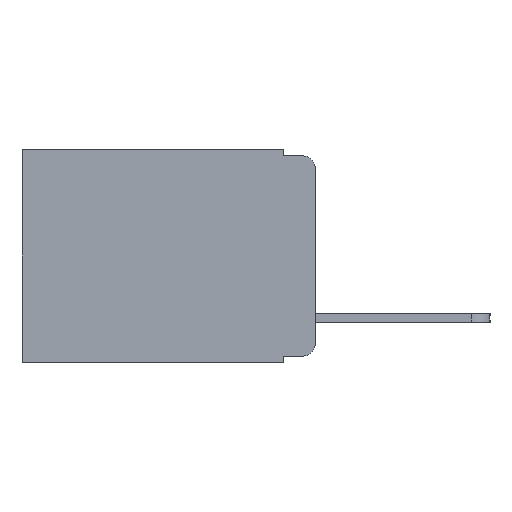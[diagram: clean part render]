
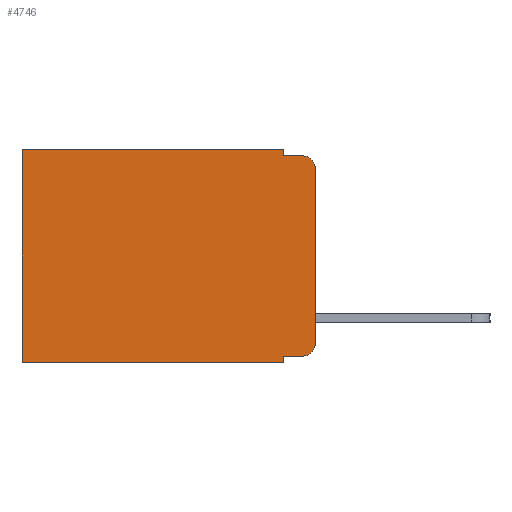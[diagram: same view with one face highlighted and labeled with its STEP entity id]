
A CAD part, left-side view. The second image highlights one B-rep face of the part: STEP entity #4746.
In plain terms, the highlighted planar face has unit normal (-1, 0, 0).
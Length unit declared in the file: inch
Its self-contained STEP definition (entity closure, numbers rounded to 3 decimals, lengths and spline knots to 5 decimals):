
#179 = CARTESIAN_POINT ( 'NONE',  ( 0.298, 0.02, -0.333 ) ) ;
#397 = EDGE_CURVE ( 'NONE', #7864, #15411, #7242, .T. ) ;
#453 = CARTESIAN_POINT ( 'NONE',  ( 0.298, 0.051, -0.333 ) ) ;
#801 = EDGE_CURVE ( 'NONE', #10526, #15889, #5974, .T. ) ;
#900 = VERTEX_POINT ( 'NONE', #15758 ) ;
#1177 = CARTESIAN_POINT ( 'NONE',  ( 0.298, 0., -0.313 ) ) ;
#1246 = VERTEX_POINT ( 'NONE', #7143 ) ;
#1386 = LINE ( 'NONE', #15184, #13645 ) ;
#1402 = CARTESIAN_POINT ( 'NONE',  ( 0.298, 0., 0. ) ) ;
#2351 = DIRECTION ( 'NONE',  ( 0., -1., 0. ) ) ;
#2799 = DIRECTION ( 'NONE',  ( 0., -1., 0. ) ) ;
#2894 = ORIENTED_EDGE ( 'NONE', *, *, #16190, .F. ) ;
#3100 = LINE ( 'NONE', #17560, #6743 ) ;
#3113 = CARTESIAN_POINT ( 'NONE',  ( 0.298, 0.051, -0.01 ) ) ;
#3884 = VERTEX_POINT ( 'NONE', #15283 ) ;
#4071 = EDGE_CURVE ( 'NONE', #10526, #7864, #5906, .T. ) ;
#4098 = CARTESIAN_POINT ( 'NONE',  ( 0.298, 0.473, 0. ) ) ;
#4107 = ORIENTED_EDGE ( 'NONE', *, *, #8979, .T. ) ;
#4514 = EDGE_LOOP ( 'NONE', ( #13406, #15881, #5519, #2894, #4107, #16439, #17451, #18480, #11206, #8338 ) ) ;
#4746 = ADVANCED_FACE ( 'NONE', ( #17765 ), #8177, .F. ) ;
#5051 = DIRECTION ( 'NONE',  ( -1., 0., 0. ) ) ;
#5519 = ORIENTED_EDGE ( 'NONE', *, *, #10094, .F. ) ;
#5906 = LINE ( 'NONE', #453, #14370 ) ;
#5921 = DIRECTION ( 'NONE',  ( 0., 0., -1. ) ) ;
#5974 = LINE ( 'NONE', #16728, #17634 ) ;
#6006 = LINE ( 'NONE', #3113, #10203 ) ;
#6701 = DIRECTION ( 'NONE',  ( 0., 1., 0. ) ) ;
#6743 = VECTOR ( 'NONE', #18883, 39.37008 ) ;
#7053 = EDGE_CURVE ( 'NONE', #15889, #7070, #11184, .T. ) ;
#7070 = VERTEX_POINT ( 'NONE', #11303 ) ;
#7143 = CARTESIAN_POINT ( 'NONE',  ( 0.298, 0.051, -0.01 ) ) ;
#7199 = AXIS2_PLACEMENT_3D ( 'NONE', #16201, #5051, #13445 ) ;
#7242 = CIRCLE ( 'NONE', #7199, 0.02 ) ;
#7453 = VERTEX_POINT ( 'NONE', #11986 ) ;
#7864 = VERTEX_POINT ( 'NONE', #179 ) ;
#8177 = PLANE ( 'NONE',  #19312 ) ;
#8287 = CARTESIAN_POINT ( 'NONE',  ( 0.298, 0.051, 0. ) ) ;
#8338 = ORIENTED_EDGE ( 'NONE', *, *, #397, .T. ) ;
#8865 = CARTESIAN_POINT ( 'NONE',  ( 0.298, 0.02, -0.03 ) ) ;
#8926 = CARTESIAN_POINT ( 'NONE',  ( 0.298, 0., 0. ) ) ;
#8979 = EDGE_CURVE ( 'NONE', #17239, #3884, #1386, .T. ) ;
#9280 = CARTESIAN_POINT ( 'NONE',  ( 0.298, 0., -0.343 ) ) ;
#9281 = DIRECTION ( 'NONE',  ( 0., 0., -1. ) ) ;
#9441 = AXIS2_PLACEMENT_3D ( 'NONE', #8865, #18719, #10402 ) ;
#10094 = EDGE_CURVE ( 'NONE', #1246, #900, #6006, .T. ) ;
#10203 = VECTOR ( 'NONE', #2351, 39.37008 ) ;
#10402 = DIRECTION ( 'NONE',  ( 0., 0., -1. ) ) ;
#10526 = VERTEX_POINT ( 'NONE', #12704 ) ;
#10699 = VECTOR ( 'NONE', #11778, 39.37008 ) ;
#11184 = LINE ( 'NONE', #9280, #10699 ) ;
#11206 = ORIENTED_EDGE ( 'NONE', *, *, #4071, .T. ) ;
#11303 = CARTESIAN_POINT ( 'NONE',  ( 0.298, 0.473, -0.343 ) ) ;
#11778 = DIRECTION ( 'NONE',  ( 0., 1., 0. ) ) ;
#11986 = CARTESIAN_POINT ( 'NONE',  ( 0.298, 0., -0.03 ) ) ;
#12704 = CARTESIAN_POINT ( 'NONE',  ( 0.298, 0.051, -0.333 ) ) ;
#12705 = CIRCLE ( 'NONE', #9441, 0.02 ) ;
#12755 = CARTESIAN_POINT ( 'NONE',  ( 0.298, 0.051, -0.343 ) ) ;
#13406 = ORIENTED_EDGE ( 'NONE', *, *, #15495, .F. ) ;
#13445 = DIRECTION ( 'NONE',  ( 0., 0., -1. ) ) ;
#13645 = VECTOR ( 'NONE', #6701, 39.37008 ) ;
#13682 = DIRECTION ( 'NONE',  ( 0., 0., -1. ) ) ;
#14370 = VECTOR ( 'NONE', #2799, 39.37008 ) ;
#15184 = CARTESIAN_POINT ( 'NONE',  ( 0.298, 0., 0. ) ) ;
#15283 = CARTESIAN_POINT ( 'NONE',  ( 0.298, 0.473, 0. ) ) ;
#15411 = VERTEX_POINT ( 'NONE', #1177 ) ;
#15495 = EDGE_CURVE ( 'NONE', #7453, #15411, #17058, .T. ) ;
#15758 = CARTESIAN_POINT ( 'NONE',  ( 0.298, 0.02, -0.01 ) ) ;
#15881 = ORIENTED_EDGE ( 'NONE', *, *, #16089, .T. ) ;
#15889 = VERTEX_POINT ( 'NONE', #12755 ) ;
#16085 = DIRECTION ( 'NONE',  ( 1., 0., 0. ) ) ;
#16089 = EDGE_CURVE ( 'NONE', #7453, #900, #12705, .T. ) ;
#16190 = EDGE_CURVE ( 'NONE', #17239, #1246, #3100, .T. ) ;
#16201 = CARTESIAN_POINT ( 'NONE',  ( 0.298, 0.02, -0.313 ) ) ;
#16439 = ORIENTED_EDGE ( 'NONE', *, *, #18828, .T. ) ;
#16673 = VECTOR ( 'NONE', #9281, 39.37008 ) ;
#16718 = VECTOR ( 'NONE', #18633, 39.37008 ) ;
#16728 = CARTESIAN_POINT ( 'NONE',  ( 0.298, 0.051, 0. ) ) ;
#17058 = LINE ( 'NONE', #1402, #16673 ) ;
#17107 = LINE ( 'NONE', #4098, #16718 ) ;
#17239 = VERTEX_POINT ( 'NONE', #8287 ) ;
#17451 = ORIENTED_EDGE ( 'NONE', *, *, #7053, .F. ) ;
#17560 = CARTESIAN_POINT ( 'NONE',  ( 0.298, 0.051, 0. ) ) ;
#17634 = VECTOR ( 'NONE', #5921, 39.37008 ) ;
#17765 = FACE_OUTER_BOUND ( 'NONE', #4514, .T. ) ;
#18480 = ORIENTED_EDGE ( 'NONE', *, *, #801, .F. ) ;
#18633 = DIRECTION ( 'NONE',  ( 0., 0., -1. ) ) ;
#18719 = DIRECTION ( 'NONE',  ( -1., 0., 0. ) ) ;
#18828 = EDGE_CURVE ( 'NONE', #3884, #7070, #17107, .T. ) ;
#18883 = DIRECTION ( 'NONE',  ( 0., 0., -1. ) ) ;
#19312 = AXIS2_PLACEMENT_3D ( 'NONE', #8926, #16085, #13682 ) ;
